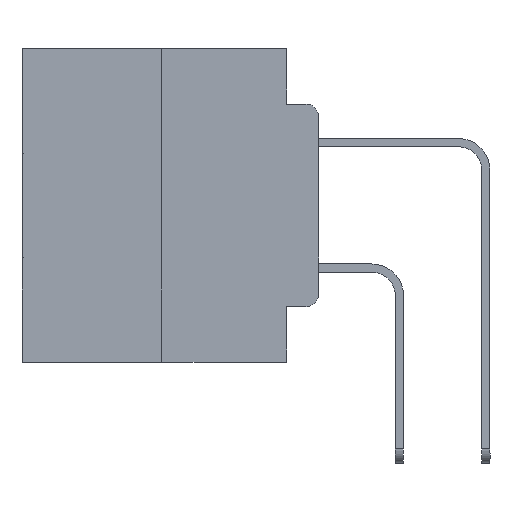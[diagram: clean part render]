
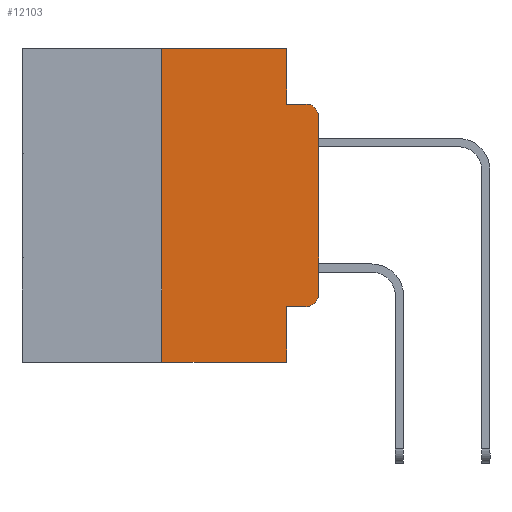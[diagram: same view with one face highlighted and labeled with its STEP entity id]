
A CAD part, left-side view. The second image highlights one B-rep face of the part: STEP entity #12103.
In plain terms, the highlighted planar face has unit normal (-1, 0, 0).
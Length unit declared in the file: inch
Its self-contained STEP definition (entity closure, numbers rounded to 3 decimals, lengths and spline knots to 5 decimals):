
#83 = CARTESIAN_POINT ( 'NONE',  ( 0., 0.473, -0.5 ) ) ;
#244 = VERTEX_POINT ( 'NONE', #24768 ) ;
#401 = ORIENTED_EDGE ( 'NONE', *, *, #20727, .T. ) ;
#408 = LINE ( 'NONE', #28228, #10212 ) ;
#698 = CIRCLE ( 'NONE', #5553, 0.02 ) ;
#788 = LINE ( 'NONE', #83, #5157 ) ;
#1649 = VECTOR ( 'NONE', #17220, 39.37008 ) ;
#2048 = CARTESIAN_POINT ( 'NONE',  ( 0., 0.473, 0. ) ) ;
#2195 = FACE_OUTER_BOUND ( 'NONE', #6527, .T. ) ;
#3029 = CARTESIAN_POINT ( 'NONE',  ( 0., 0.25, 0. ) ) ;
#5126 = VERTEX_POINT ( 'NONE', #16039 ) ;
#5157 = VECTOR ( 'NONE', #26331, 39.37008 ) ;
#5373 = CARTESIAN_POINT ( 'NONE',  ( 0., 0.473, 0. ) ) ;
#5553 = AXIS2_PLACEMENT_3D ( 'NONE', #11329, #9038, #6900 ) ;
#5664 = VECTOR ( 'NONE', #12309, 39.37008 ) ;
#6228 = ORIENTED_EDGE ( 'NONE', *, *, #18357, .T. ) ;
#6527 = EDGE_LOOP ( 'NONE', ( #20685, #401, #10287, #15292, #20124, #17212, #24454, #28399, #6228, #20729 ) ) ;
#6900 = DIRECTION ( 'NONE',  ( 0., 0., -1. ) ) ;
#6905 = CIRCLE ( 'NONE', #26340, 0.02 ) ;
#7327 = LINE ( 'NONE', #21175, #7899 ) ;
#7899 = VECTOR ( 'NONE', #14030, 39.37008 ) ;
#8007 = VERTEX_POINT ( 'NONE', #12324 ) ;
#8277 = CARTESIAN_POINT ( 'NONE',  ( 0., 0.051, -0.4115 ) ) ;
#9038 = DIRECTION ( 'NONE',  ( -1., 0., 0. ) ) ;
#9052 = CARTESIAN_POINT ( 'NONE',  ( 0., 0.051, 0. ) ) ;
#10212 = VECTOR ( 'NONE', #28815, 39.37008 ) ;
#10243 = DIRECTION ( 'NONE',  ( 0., -1., 0. ) ) ;
#10287 = ORIENTED_EDGE ( 'NONE', *, *, #22703, .F. ) ;
#10372 = VERTEX_POINT ( 'NONE', #13448 ) ;
#10998 = VECTOR ( 'NONE', #20781, 39.37008 ) ;
#11242 = CARTESIAN_POINT ( 'NONE',  ( 0., 0.25, -0.5 ) ) ;
#11329 = CARTESIAN_POINT ( 'NONE',  ( 0., 0.02, -0.3915 ) ) ;
#12103 = ADVANCED_FACE ( 'NONE', ( #2195 ), #20742, .F. ) ;
#12104 = EDGE_CURVE ( 'NONE', #10372, #8007, #698, .T. ) ;
#12309 = DIRECTION ( 'NONE',  ( 0., 0., 1. ) ) ;
#12324 = CARTESIAN_POINT ( 'NONE',  ( 0., 0., -0.3915 ) ) ;
#12613 = VERTEX_POINT ( 'NONE', #18700 ) ;
#13435 = VECTOR ( 'NONE', #10243, 39.37008 ) ;
#13448 = CARTESIAN_POINT ( 'NONE',  ( 0., 0.02, -0.4115 ) ) ;
#13800 = AXIS2_PLACEMENT_3D ( 'NONE', #2048, #22868, #25756 ) ;
#13934 = CARTESIAN_POINT ( 'NONE',  ( 0., 0., 0. ) ) ;
#14030 = DIRECTION ( 'NONE',  ( 0., -1., 0. ) ) ;
#14578 = CARTESIAN_POINT ( 'NONE',  ( 0., 0.051, -0.5 ) ) ;
#15292 = ORIENTED_EDGE ( 'NONE', *, *, #20770, .F. ) ;
#15433 = EDGE_CURVE ( 'NONE', #16377, #16147, #788, .T. ) ;
#15931 = CARTESIAN_POINT ( 'NONE',  ( 0., 0., -0.1085 ) ) ;
#16039 = CARTESIAN_POINT ( 'NONE',  ( 0., 0.25, 0. ) ) ;
#16147 = VERTEX_POINT ( 'NONE', #14578 ) ;
#16377 = VERTEX_POINT ( 'NONE', #11242 ) ;
#17212 = ORIENTED_EDGE ( 'NONE', *, *, #28026, .F. ) ;
#17220 = DIRECTION ( 'NONE',  ( 0., 0., -1. ) ) ;
#17542 = CARTESIAN_POINT ( 'NONE',  ( 0., 0.051, 0. ) ) ;
#18011 = DIRECTION ( 'NONE',  ( -1., 0., 0. ) ) ;
#18357 = EDGE_CURVE ( 'NONE', #26783, #10372, #408, .T. ) ;
#18700 = CARTESIAN_POINT ( 'NONE',  ( 0., 0.051, -0.0885 ) ) ;
#18776 = LINE ( 'NONE', #13934, #10998 ) ;
#20124 = ORIENTED_EDGE ( 'NONE', *, *, #28471, .F. ) ;
#20444 = DIRECTION ( 'NONE',  ( 0., 0., -1. ) ) ;
#20685 = ORIENTED_EDGE ( 'NONE', *, *, #26387, .T. ) ;
#20727 = EDGE_CURVE ( 'NONE', #29404, #244, #6905, .T. ) ;
#20729 = ORIENTED_EDGE ( 'NONE', *, *, #12104, .T. ) ;
#20742 = PLANE ( 'NONE',  #13800 ) ;
#20770 = EDGE_CURVE ( 'NONE', #22393, #12613, #25016, .T. ) ;
#20781 = DIRECTION ( 'NONE',  ( 0., 0., 1. ) ) ;
#21175 = CARTESIAN_POINT ( 'NONE',  ( 0., 0.051, -0.0885 ) ) ;
#21967 = VECTOR ( 'NONE', #20444, 39.37008 ) ;
#22393 = VERTEX_POINT ( 'NONE', #17542 ) ;
#22570 = CARTESIAN_POINT ( 'NONE',  ( 0., 0.02, -0.1085 ) ) ;
#22703 = EDGE_CURVE ( 'NONE', #12613, #244, #7327, .T. ) ;
#22868 = DIRECTION ( 'NONE',  ( 1., 0., 0. ) ) ;
#23384 = LINE ( 'NONE', #3029, #5664 ) ;
#24113 = EDGE_CURVE ( 'NONE', #26783, #16147, #24357, .T. ) ;
#24357 = LINE ( 'NONE', #24655, #1649 ) ;
#24454 = ORIENTED_EDGE ( 'NONE', *, *, #15433, .T. ) ;
#24655 = CARTESIAN_POINT ( 'NONE',  ( 0., 0.051, 0. ) ) ;
#24768 = CARTESIAN_POINT ( 'NONE',  ( 0., 0.02, -0.0885 ) ) ;
#25016 = LINE ( 'NONE', #9052, #21967 ) ;
#25756 = DIRECTION ( 'NONE',  ( 0., 0., -1. ) ) ;
#26213 = LINE ( 'NONE', #5373, #13435 ) ;
#26331 = DIRECTION ( 'NONE',  ( 0., -1., 0. ) ) ;
#26340 = AXIS2_PLACEMENT_3D ( 'NONE', #22570, #18011, #29444 ) ;
#26387 = EDGE_CURVE ( 'NONE', #8007, #29404, #18776, .T. ) ;
#26783 = VERTEX_POINT ( 'NONE', #8277 ) ;
#28026 = EDGE_CURVE ( 'NONE', #16377, #5126, #23384, .T. ) ;
#28228 = CARTESIAN_POINT ( 'NONE',  ( 0., 0.051, -0.4115 ) ) ;
#28399 = ORIENTED_EDGE ( 'NONE', *, *, #24113, .F. ) ;
#28471 = EDGE_CURVE ( 'NONE', #5126, #22393, #26213, .T. ) ;
#28815 = DIRECTION ( 'NONE',  ( 0., -1., 0. ) ) ;
#29404 = VERTEX_POINT ( 'NONE', #15931 ) ;
#29444 = DIRECTION ( 'NONE',  ( 0., 0., -1. ) ) ;
